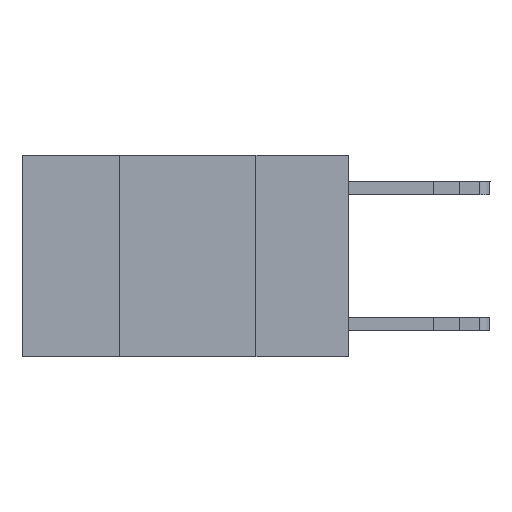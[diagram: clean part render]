
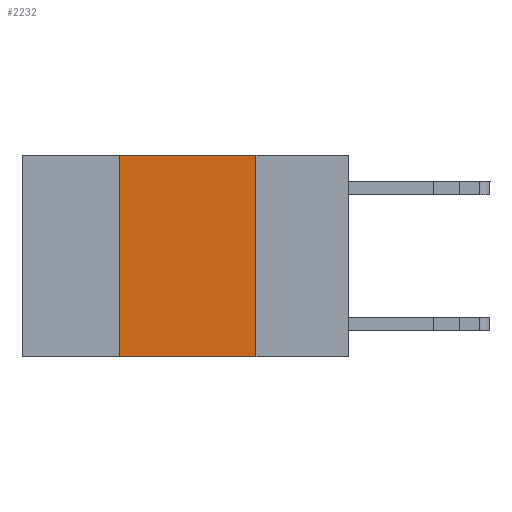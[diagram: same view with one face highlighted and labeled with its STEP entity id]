
A CAD part, left-side view. The second image highlights one B-rep face of the part: STEP entity #2232.
In plain terms, the highlighted planar face has unit normal (-1, 0, 0).
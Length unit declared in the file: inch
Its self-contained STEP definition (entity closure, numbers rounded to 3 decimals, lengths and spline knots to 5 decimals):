
#343 = VERTEX_POINT ( 'NONE', #2924 ) ;
#691 = EDGE_CURVE ( 'NONE', #8904, #11895, #13462, .T. ) ;
#2232 = ADVANCED_FACE ( 'NONE', ( #8959 ), #4920, .F. ) ;
#2792 = EDGE_CURVE ( 'NONE', #343, #3100, #17715, .T. ) ;
#2924 = CARTESIAN_POINT ( 'NONE',  ( 0., 0.42, -0.37 ) ) ;
#3057 = LINE ( 'NONE', #8382, #6930 ) ;
#3077 = ORIENTED_EDGE ( 'NONE', *, *, #10013, .F. ) ;
#3100 = VERTEX_POINT ( 'NONE', #10124 ) ;
#3535 = DIRECTION ( 'NONE',  ( 0., 0., -1. ) ) ;
#4841 = EDGE_LOOP ( 'NONE', ( #17738, #6589, #3077, #13365 ) ) ;
#4920 = PLANE ( 'NONE',  #13747 ) ;
#6108 = CARTESIAN_POINT ( 'NONE',  ( 0., 0.6, -0.37 ) ) ;
#6573 = DIRECTION ( 'NONE',  ( 1., 0., 0. ) ) ;
#6589 = ORIENTED_EDGE ( 'NONE', *, *, #691, .F. ) ;
#6930 = VECTOR ( 'NONE', #11321, 39.37008 ) ;
#7509 = EDGE_CURVE ( 'NONE', #11895, #3100, #16431, .T. ) ;
#8142 = CARTESIAN_POINT ( 'NONE',  ( 0., 0.6, 0. ) ) ;
#8382 = CARTESIAN_POINT ( 'NONE',  ( 0., 0.42, 0. ) ) ;
#8904 = VERTEX_POINT ( 'NONE', #13716 ) ;
#8959 = FACE_OUTER_BOUND ( 'NONE', #4841, .T. ) ;
#9753 = VECTOR ( 'NONE', #12167, 39.37008 ) ;
#10013 = EDGE_CURVE ( 'NONE', #343, #8904, #3057, .T. ) ;
#10124 = CARTESIAN_POINT ( 'NONE',  ( 0., 0.17, -0.37 ) ) ;
#10323 = VECTOR ( 'NONE', #11682, 39.37008 ) ;
#10772 = CARTESIAN_POINT ( 'NONE',  ( 0., 0.17, 0. ) ) ;
#11321 = DIRECTION ( 'NONE',  ( 0., 0., 1. ) ) ;
#11682 = DIRECTION ( 'NONE',  ( 0., -1., 0. ) ) ;
#11895 = VERTEX_POINT ( 'NONE', #17234 ) ;
#12167 = DIRECTION ( 'NONE',  ( 0., -1., 0. ) ) ;
#13365 = ORIENTED_EDGE ( 'NONE', *, *, #2792, .T. ) ;
#13462 = LINE ( 'NONE', #8142, #9753 ) ;
#13716 = CARTESIAN_POINT ( 'NONE',  ( 0., 0.42, 0. ) ) ;
#13747 = AXIS2_PLACEMENT_3D ( 'NONE', #14944, #6573, #3535 ) ;
#14944 = CARTESIAN_POINT ( 'NONE',  ( 0., 0.6, 0. ) ) ;
#15112 = DIRECTION ( 'NONE',  ( 0., 0., -1. ) ) ;
#16431 = LINE ( 'NONE', #10772, #17465 ) ;
#17234 = CARTESIAN_POINT ( 'NONE',  ( 0., 0.17, 0. ) ) ;
#17465 = VECTOR ( 'NONE', #15112, 39.37008 ) ;
#17715 = LINE ( 'NONE', #6108, #10323 ) ;
#17738 = ORIENTED_EDGE ( 'NONE', *, *, #7509, .F. ) ;
